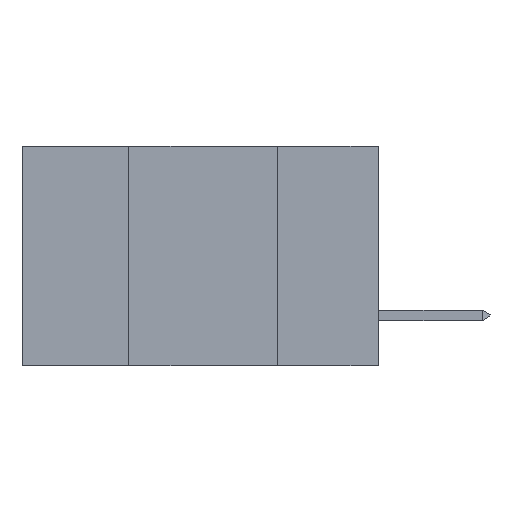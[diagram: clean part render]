
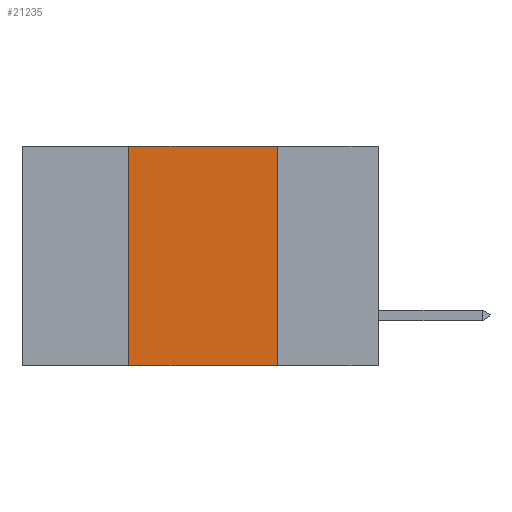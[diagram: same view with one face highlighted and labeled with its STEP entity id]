
A CAD part, left-side view. The second image highlights one B-rep face of the part: STEP entity #21235.
In plain terms, the highlighted planar face has unit normal (-1, 0, 0).
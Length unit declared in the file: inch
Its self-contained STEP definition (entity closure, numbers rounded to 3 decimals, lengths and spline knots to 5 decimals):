
#43 = EDGE_CURVE ( 'NONE', #17084, #13668, #17994, .T. ) ;
#201 = CARTESIAN_POINT ( 'NONE',  ( 0., 0.6, 0. ) ) ;
#309 = DIRECTION ( 'NONE',  ( 0., 0., -1. ) ) ;
#1714 = CARTESIAN_POINT ( 'NONE',  ( 0., 0.6, -0.37 ) ) ;
#3443 = VECTOR ( 'NONE', #12497, 39.37008 ) ;
#3699 = LINE ( 'NONE', #17637, #3443 ) ;
#4511 = AXIS2_PLACEMENT_3D ( 'NONE', #201, #5444, #309 ) ;
#5058 = LINE ( 'NONE', #10661, #10701 ) ;
#5159 = CARTESIAN_POINT ( 'NONE',  ( 0., 0.42, 0. ) ) ;
#5444 = DIRECTION ( 'NONE',  ( 1., 0., 0. ) ) ;
#5878 = DIRECTION ( 'NONE',  ( 0., -1., 0. ) ) ;
#6879 = EDGE_CURVE ( 'NONE', #8710, #17084, #5058, .T. ) ;
#7010 = VECTOR ( 'NONE', #15332, 39.37008 ) ;
#7549 = CARTESIAN_POINT ( 'NONE',  ( 0., 0.17, 0. ) ) ;
#8710 = VERTEX_POINT ( 'NONE', #17113 ) ;
#9134 = ORIENTED_EDGE ( 'NONE', *, *, #19037, .T. ) ;
#10567 = CARTESIAN_POINT ( 'NONE',  ( 0., 0.17, -0.37 ) ) ;
#10661 = CARTESIAN_POINT ( 'NONE',  ( 0., 0.42, -0.37 ) ) ;
#10701 = VECTOR ( 'NONE', #17617, 39.37008 ) ;
#11090 = EDGE_LOOP ( 'NONE', ( #14632, #13302, #19296, #9134 ) ) ;
#11340 = VERTEX_POINT ( 'NONE', #10567 ) ;
#12497 = DIRECTION ( 'NONE',  ( 0., 0., -1. ) ) ;
#13302 = ORIENTED_EDGE ( 'NONE', *, *, #43, .F. ) ;
#13668 = VERTEX_POINT ( 'NONE', #7549 ) ;
#13898 = FACE_OUTER_BOUND ( 'NONE', #11090, .T. ) ;
#14632 = ORIENTED_EDGE ( 'NONE', *, *, #21786, .F. ) ;
#14906 = VECTOR ( 'NONE', #5878, 39.37008 ) ;
#15332 = DIRECTION ( 'NONE',  ( 0., -1., 0. ) ) ;
#17045 = LINE ( 'NONE', #1714, #7010 ) ;
#17084 = VERTEX_POINT ( 'NONE', #5159 ) ;
#17113 = CARTESIAN_POINT ( 'NONE',  ( 0., 0.42, -0.37 ) ) ;
#17617 = DIRECTION ( 'NONE',  ( 0., 0., 1. ) ) ;
#17637 = CARTESIAN_POINT ( 'NONE',  ( 0., 0.17, -0.37 ) ) ;
#17890 = PLANE ( 'NONE',  #4511 ) ;
#17994 = LINE ( 'NONE', #21864, #14906 ) ;
#19037 = EDGE_CURVE ( 'NONE', #8710, #11340, #17045, .T. ) ;
#19296 = ORIENTED_EDGE ( 'NONE', *, *, #6879, .F. ) ;
#21235 = ADVANCED_FACE ( 'NONE', ( #13898 ), #17890, .F. ) ;
#21786 = EDGE_CURVE ( 'NONE', #13668, #11340, #3699, .T. ) ;
#21864 = CARTESIAN_POINT ( 'NONE',  ( 0., 0.6, 0. ) ) ;
